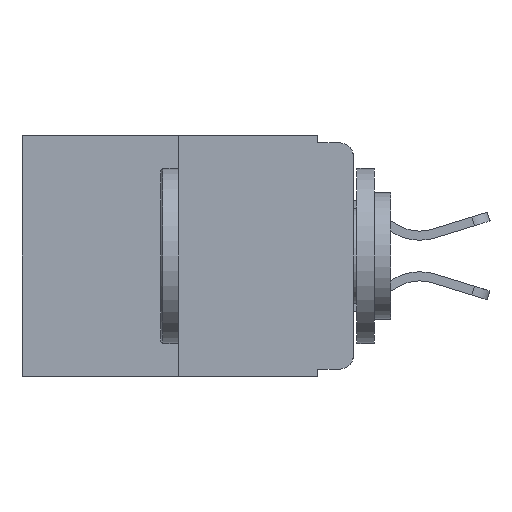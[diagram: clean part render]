
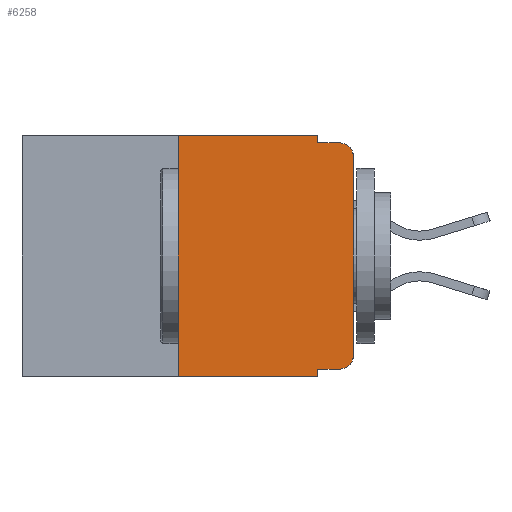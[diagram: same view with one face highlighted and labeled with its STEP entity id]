
A CAD part, left-side view. The second image highlights one B-rep face of the part: STEP entity #6258.
In plain terms, the highlighted planar face has unit normal (-1, 0, 0).
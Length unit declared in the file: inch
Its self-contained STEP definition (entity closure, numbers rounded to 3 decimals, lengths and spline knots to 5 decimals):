
#57 = ORIENTED_EDGE ( 'NONE', *, *, #6120, .F. ) ;
#111 = VECTOR ( 'NONE', #7425, 39.37008 ) ;
#677 = ORIENTED_EDGE ( 'NONE', *, *, #9745, .F. ) ;
#1161 = DIRECTION ( 'NONE',  ( 0., -1., 0. ) ) ;
#1178 = VERTEX_POINT ( 'NONE', #24450 ) ;
#1406 = EDGE_CURVE ( 'NONE', #1178, #21627, #10189, .T. ) ;
#1681 = EDGE_CURVE ( 'NONE', #23739, #15669, #9881, .T. ) ;
#1707 = DIRECTION ( 'NONE',  ( -1., 0., 0. ) ) ;
#2747 = VECTOR ( 'NONE', #24528, 39.37008 ) ;
#2808 = ORIENTED_EDGE ( 'NONE', *, *, #6850, .T. ) ;
#3254 = VERTEX_POINT ( 'NONE', #22708 ) ;
#3613 = CARTESIAN_POINT ( 'NONE',  ( 0., 0.051, 0. ) ) ;
#3986 = LINE ( 'NONE', #3613, #25110 ) ;
#3992 = ORIENTED_EDGE ( 'NONE', *, *, #24903, .F. ) ;
#4131 = EDGE_CURVE ( 'NONE', #17995, #1178, #22922, .T. ) ;
#4291 = CARTESIAN_POINT ( 'NONE',  ( 0., 0.473, -0.343 ) ) ;
#6120 = EDGE_CURVE ( 'NONE', #3254, #21463, #3986, .T. ) ;
#6146 = CARTESIAN_POINT ( 'NONE',  ( 0., 0., -0.313 ) ) ;
#6258 = ADVANCED_FACE ( 'NONE', ( #16078 ), #13916, .F. ) ;
#6526 = CARTESIAN_POINT ( 'NONE',  ( 0., 0.051, -0.333 ) ) ;
#6850 = EDGE_CURVE ( 'NONE', #22013, #10519, #17630, .T. ) ;
#7425 = DIRECTION ( 'NONE',  ( 0., 0., 1. ) ) ;
#7596 = CARTESIAN_POINT ( 'NONE',  ( 0., 0.051, 0. ) ) ;
#8018 = DIRECTION ( 'NONE',  ( 1., 0., 0. ) ) ;
#8125 = VECTOR ( 'NONE', #21247, 39.37008 ) ;
#8492 = CARTESIAN_POINT ( 'NONE',  ( 0., 0., 0. ) ) ;
#8742 = LINE ( 'NONE', #17270, #8125 ) ;
#8836 = CIRCLE ( 'NONE', #25007, 0.02 ) ;
#9111 = LINE ( 'NONE', #25042, #13792 ) ;
#9745 = EDGE_CURVE ( 'NONE', #13264, #3254, #9111, .T. ) ;
#9881 = LINE ( 'NONE', #19227, #15170 ) ;
#9956 = CARTESIAN_POINT ( 'NONE',  ( 0., 0.02, -0.333 ) ) ;
#10189 = CIRCLE ( 'NONE', #10959, 0.02 ) ;
#10519 = VERTEX_POINT ( 'NONE', #19674 ) ;
#10959 = AXIS2_PLACEMENT_3D ( 'NONE', #11913, #19812, #19782 ) ;
#11913 = CARTESIAN_POINT ( 'NONE',  ( 0., 0.02, -0.03 ) ) ;
#13264 = VERTEX_POINT ( 'NONE', #23637 ) ;
#13648 = CARTESIAN_POINT ( 'NONE',  ( 0., 0.02, -0.313 ) ) ;
#13792 = VECTOR ( 'NONE', #1161, 39.37008 ) ;
#13915 = DIRECTION ( 'NONE',  ( 0., -1., 0. ) ) ;
#13916 = PLANE ( 'NONE',  #21854 ) ;
#15170 = VECTOR ( 'NONE', #13915, 39.37008 ) ;
#15267 = EDGE_CURVE ( 'NONE', #21463, #21627, #8742, .T. ) ;
#15337 = CARTESIAN_POINT ( 'NONE',  ( 0., 0.25, 0. ) ) ;
#15391 = EDGE_CURVE ( 'NONE', #23739, #10519, #15615, .T. ) ;
#15615 = LINE ( 'NONE', #7596, #20960 ) ;
#15669 = VERTEX_POINT ( 'NONE', #9956 ) ;
#16078 = FACE_OUTER_BOUND ( 'NONE', #20382, .T. ) ;
#16152 = ORIENTED_EDGE ( 'NONE', *, *, #4131, .T. ) ;
#16859 = EDGE_CURVE ( 'NONE', #15669, #17995, #8836, .T. ) ;
#17066 = CARTESIAN_POINT ( 'NONE',  ( 0., 0.25, -0.343 ) ) ;
#17270 = CARTESIAN_POINT ( 'NONE',  ( 0., 0.051, -0.01 ) ) ;
#17271 = ORIENTED_EDGE ( 'NONE', *, *, #16859, .T. ) ;
#17466 = CARTESIAN_POINT ( 'NONE',  ( 0., 0.051, -0.01 ) ) ;
#17524 = DIRECTION ( 'NONE',  ( 0., 0., -1. ) ) ;
#17630 = LINE ( 'NONE', #4291, #18246 ) ;
#17995 = VERTEX_POINT ( 'NONE', #6146 ) ;
#18035 = ORIENTED_EDGE ( 'NONE', *, *, #1681, .T. ) ;
#18197 = DIRECTION ( 'NONE',  ( 0., -1., 0. ) ) ;
#18246 = VECTOR ( 'NONE', #18197, 39.37008 ) ;
#18441 = ORIENTED_EDGE ( 'NONE', *, *, #15391, .F. ) ;
#18725 = ORIENTED_EDGE ( 'NONE', *, *, #1406, .T. ) ;
#19227 = CARTESIAN_POINT ( 'NONE',  ( 0., 0.051, -0.333 ) ) ;
#19674 = CARTESIAN_POINT ( 'NONE',  ( 0., 0.051, -0.343 ) ) ;
#19782 = DIRECTION ( 'NONE',  ( 0., 0., -1. ) ) ;
#19812 = DIRECTION ( 'NONE',  ( -1., 0., 0. ) ) ;
#20382 = EDGE_LOOP ( 'NONE', ( #16152, #18725, #20788, #57, #677, #3992, #2808, #18441, #18035, #17271 ) ) ;
#20385 = DIRECTION ( 'NONE',  ( 0., 0., -1. ) ) ;
#20788 = ORIENTED_EDGE ( 'NONE', *, *, #15267, .F. ) ;
#20960 = VECTOR ( 'NONE', #23573, 39.37008 ) ;
#21247 = DIRECTION ( 'NONE',  ( 0., -1., 0. ) ) ;
#21463 = VERTEX_POINT ( 'NONE', #17466 ) ;
#21627 = VERTEX_POINT ( 'NONE', #22039 ) ;
#21854 = AXIS2_PLACEMENT_3D ( 'NONE', #25801, #8018, #22015 ) ;
#22013 = VERTEX_POINT ( 'NONE', #17066 ) ;
#22015 = DIRECTION ( 'NONE',  ( 0., 0., -1. ) ) ;
#22039 = CARTESIAN_POINT ( 'NONE',  ( 0., 0.02, -0.01 ) ) ;
#22103 = LINE ( 'NONE', #15337, #111 ) ;
#22708 = CARTESIAN_POINT ( 'NONE',  ( 0., 0.051, 0. ) ) ;
#22922 = LINE ( 'NONE', #8492, #2747 ) ;
#23573 = DIRECTION ( 'NONE',  ( 0., 0., -1. ) ) ;
#23637 = CARTESIAN_POINT ( 'NONE',  ( 0., 0.25, 0. ) ) ;
#23739 = VERTEX_POINT ( 'NONE', #6526 ) ;
#24450 = CARTESIAN_POINT ( 'NONE',  ( 0., 0., -0.03 ) ) ;
#24528 = DIRECTION ( 'NONE',  ( 0., 0., 1. ) ) ;
#24903 = EDGE_CURVE ( 'NONE', #22013, #13264, #22103, .T. ) ;
#25007 = AXIS2_PLACEMENT_3D ( 'NONE', #13648, #1707, #20385 ) ;
#25042 = CARTESIAN_POINT ( 'NONE',  ( 0., 0.473, 0. ) ) ;
#25110 = VECTOR ( 'NONE', #17524, 39.37008 ) ;
#25801 = CARTESIAN_POINT ( 'NONE',  ( 0., 0.473, 0. ) ) ;
